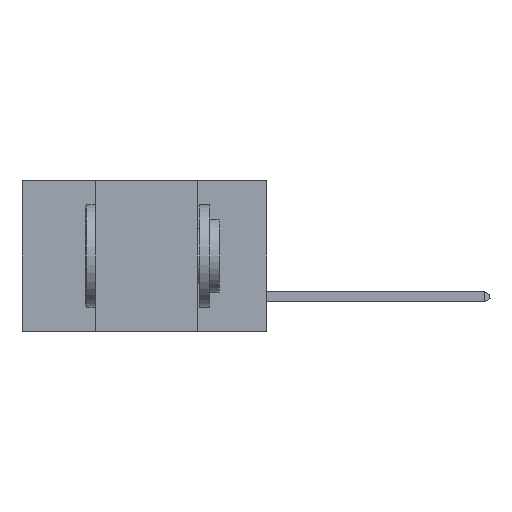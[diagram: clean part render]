
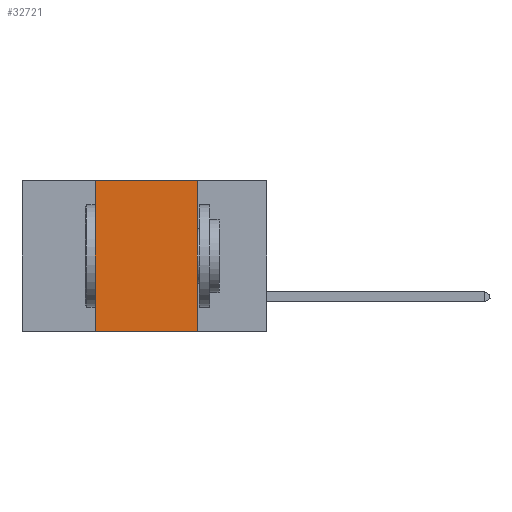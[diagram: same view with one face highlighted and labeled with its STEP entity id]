
A CAD part, left-side view. The second image highlights one B-rep face of the part: STEP entity #32721.
In plain terms, the highlighted planar face has unit normal (-1, 0, 0).
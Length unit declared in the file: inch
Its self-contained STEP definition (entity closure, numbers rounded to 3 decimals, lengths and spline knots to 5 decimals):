
#25 = VERTEX_POINT ( 'NONE', #31174 ) ;
#1780 = VERTEX_POINT ( 'NONE', #23646 ) ;
#2142 = EDGE_CURVE ( 'NONE', #4666, #25, #34306, .T. ) ;
#3428 = VECTOR ( 'NONE', #23640, 39.37008 ) ;
#4666 = VERTEX_POINT ( 'NONE', #12864 ) ;
#5154 = VECTOR ( 'NONE', #5965, 39.37008 ) ;
#5155 = LINE ( 'NONE', #23291, #3428 ) ;
#5782 = ORIENTED_EDGE ( 'NONE', *, *, #2142, .F. ) ;
#5965 = DIRECTION ( 'NONE',  ( 0., 0., 1. ) ) ;
#7088 = DIRECTION ( 'NONE',  ( 1., 0., 0. ) ) ;
#9212 = LINE ( 'NONE', #29096, #12209 ) ;
#12209 = VECTOR ( 'NONE', #34617, 39.37008 ) ;
#12864 = CARTESIAN_POINT ( 'NONE',  ( 0., 0.42, -0.37 ) ) ;
#13436 = VERTEX_POINT ( 'NONE', #32777 ) ;
#14703 = ORIENTED_EDGE ( 'NONE', *, *, #16547, .F. ) ;
#15232 = PLANE ( 'NONE',  #18623 ) ;
#15257 = VECTOR ( 'NONE', #33718, 39.37008 ) ;
#16032 = ORIENTED_EDGE ( 'NONE', *, *, #34401, .F. ) ;
#16547 = EDGE_CURVE ( 'NONE', #13436, #1780, #5155, .T. ) ;
#18623 = AXIS2_PLACEMENT_3D ( 'NONE', #29358, #7088, #23875 ) ;
#23056 = CARTESIAN_POINT ( 'NONE',  ( 0., 0.6, 0. ) ) ;
#23291 = CARTESIAN_POINT ( 'NONE',  ( 0., 0.17, 0. ) ) ;
#23640 = DIRECTION ( 'NONE',  ( 0., 0., -1. ) ) ;
#23646 = CARTESIAN_POINT ( 'NONE',  ( 0., 0.17, -0.37 ) ) ;
#23875 = DIRECTION ( 'NONE',  ( 0., 0., -1. ) ) ;
#24177 = EDGE_LOOP ( 'NONE', ( #14703, #16032, #5782, #32259 ) ) ;
#27834 = EDGE_CURVE ( 'NONE', #4666, #1780, #9212, .T. ) ;
#28510 = LINE ( 'NONE', #23056, #15257 ) ;
#29096 = CARTESIAN_POINT ( 'NONE',  ( 0., 0.6, -0.37 ) ) ;
#29358 = CARTESIAN_POINT ( 'NONE',  ( 0., 0.6, 0. ) ) ;
#30739 = FACE_OUTER_BOUND ( 'NONE', #24177, .T. ) ;
#30885 = CARTESIAN_POINT ( 'NONE',  ( 0., 0.42, 0. ) ) ;
#31174 = CARTESIAN_POINT ( 'NONE',  ( 0., 0.42, 0. ) ) ;
#32259 = ORIENTED_EDGE ( 'NONE', *, *, #27834, .T. ) ;
#32721 = ADVANCED_FACE ( 'NONE', ( #30739 ), #15232, .F. ) ;
#32777 = CARTESIAN_POINT ( 'NONE',  ( 0., 0.17, 0. ) ) ;
#33718 = DIRECTION ( 'NONE',  ( 0., -1., 0. ) ) ;
#34306 = LINE ( 'NONE', #30885, #5154 ) ;
#34401 = EDGE_CURVE ( 'NONE', #25, #13436, #28510, .T. ) ;
#34617 = DIRECTION ( 'NONE',  ( 0., -1., 0. ) ) ;
